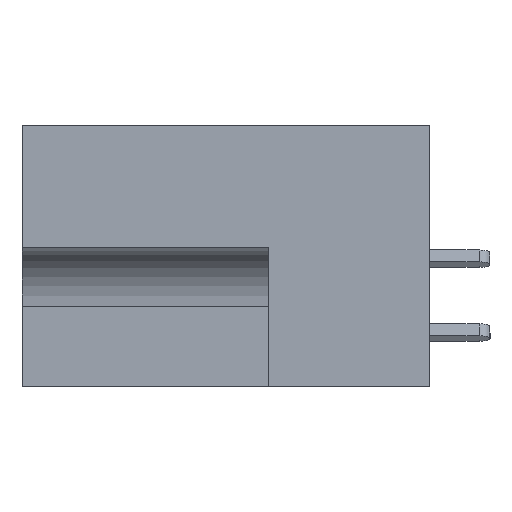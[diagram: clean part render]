
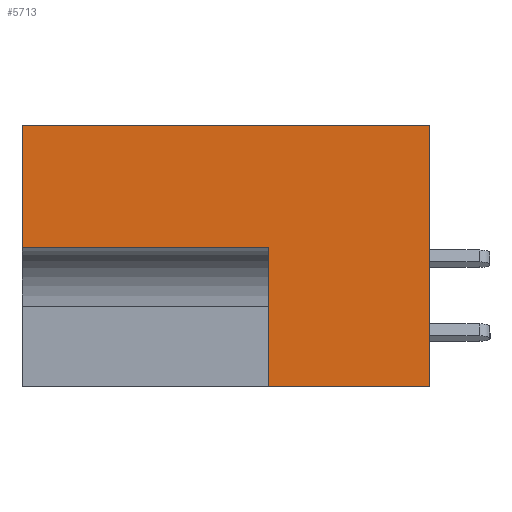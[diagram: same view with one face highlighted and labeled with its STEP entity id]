
A CAD part, left-side view. The second image highlights one B-rep face of the part: STEP entity #5713.
In plain terms, the highlighted planar face has unit normal (-1, 0, 0).
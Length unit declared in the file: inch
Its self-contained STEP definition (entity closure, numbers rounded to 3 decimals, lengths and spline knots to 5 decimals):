
#639 = CARTESIAN_POINT ( 'NONE',  ( 0., 0.453, 0. ) ) ;
#872 = AXIS2_PLACEMENT_3D ( 'NONE', #13198, #6765, #5281 ) ;
#1034 = DIRECTION ( 'NONE',  ( 0., -1., 0. ) ) ;
#1249 = DIRECTION ( 'NONE',  ( 0., 1., 0. ) ) ;
#1355 = ORIENTED_EDGE ( 'NONE', *, *, #11278, .T. ) ;
#2337 = EDGE_CURVE ( 'NONE', #8009, #20477, #3827, .T. ) ;
#2686 = CARTESIAN_POINT ( 'NONE',  ( 0., 0.328, -0.248 ) ) ;
#3179 = VERTEX_POINT ( 'NONE', #6458 ) ;
#3827 = LINE ( 'NONE', #639, #5066 ) ;
#4107 = EDGE_CURVE ( 'NONE', #3179, #8009, #11041, .T. ) ;
#4432 = ORIENTED_EDGE ( 'NONE', *, *, #12451, .F. ) ;
#4786 = EDGE_CURVE ( 'NONE', #13061, #18036, #16835, .T. ) ;
#5066 = VECTOR ( 'NONE', #8846, 39.37008 ) ;
#5281 = DIRECTION ( 'NONE',  ( 0., 0., -1. ) ) ;
#5713 = ADVANCED_FACE ( 'NONE', ( #11478 ), #16769, .F. ) ;
#5969 = VECTOR ( 'NONE', #18970, 39.37008 ) ;
#6180 = CARTESIAN_POINT ( 'NONE',  ( 0., 0.828, 0. ) ) ;
#6458 = CARTESIAN_POINT ( 'NONE',  ( 0., 0.828, -0.248 ) ) ;
#6765 = DIRECTION ( 'NONE',  ( 1., 0., 0. ) ) ;
#6984 = DIRECTION ( 'NONE',  ( 0., 0., 1. ) ) ;
#7018 = CARTESIAN_POINT ( 'NONE',  ( 0., 0., 0. ) ) ;
#7484 = CARTESIAN_POINT ( 'NONE',  ( 0., 0.453, -0.531 ) ) ;
#7502 = LINE ( 'NONE', #19053, #10277 ) ;
#7766 = CARTESIAN_POINT ( 'NONE',  ( 0., 0.328, -0.531 ) ) ;
#8009 = VERTEX_POINT ( 'NONE', #20684 ) ;
#8181 = ORIENTED_EDGE ( 'NONE', *, *, #4786, .F. ) ;
#8846 = DIRECTION ( 'NONE',  ( 0., -1., 0. ) ) ;
#9139 = EDGE_CURVE ( 'NONE', #14839, #20477, #16411, .T. ) ;
#10277 = VECTOR ( 'NONE', #1249, 39.37008 ) ;
#10609 = ORIENTED_EDGE ( 'NONE', *, *, #9139, .T. ) ;
#11041 = LINE ( 'NONE', #6180, #5969 ) ;
#11278 = EDGE_CURVE ( 'NONE', #13061, #14839, #12131, .T. ) ;
#11478 = FACE_OUTER_BOUND ( 'NONE', #19828, .T. ) ;
#12131 = LINE ( 'NONE', #7484, #13376 ) ;
#12451 = EDGE_CURVE ( 'NONE', #18036, #3179, #7502, .T. ) ;
#13061 = VERTEX_POINT ( 'NONE', #7766 ) ;
#13198 = CARTESIAN_POINT ( 'NONE',  ( 0., 0.453, 0. ) ) ;
#13294 = ORIENTED_EDGE ( 'NONE', *, *, #2337, .F. ) ;
#13298 = ORIENTED_EDGE ( 'NONE', *, *, #4107, .F. ) ;
#13376 = VECTOR ( 'NONE', #1034, 39.37008 ) ;
#14839 = VERTEX_POINT ( 'NONE', #19269 ) ;
#15191 = DIRECTION ( 'NONE',  ( 0., 0., 1. ) ) ;
#15830 = VECTOR ( 'NONE', #6984, 39.37008 ) ;
#16411 = LINE ( 'NONE', #18373, #17946 ) ;
#16769 = PLANE ( 'NONE',  #872 ) ;
#16835 = LINE ( 'NONE', #19639, #15830 ) ;
#17946 = VECTOR ( 'NONE', #15191, 39.37008 ) ;
#18036 = VERTEX_POINT ( 'NONE', #2686 ) ;
#18373 = CARTESIAN_POINT ( 'NONE',  ( 0., 0., 0. ) ) ;
#18970 = DIRECTION ( 'NONE',  ( 0., 0., 1. ) ) ;
#19053 = CARTESIAN_POINT ( 'NONE',  ( 0., 0.328, -0.248 ) ) ;
#19269 = CARTESIAN_POINT ( 'NONE',  ( 0., 0., -0.531 ) ) ;
#19639 = CARTESIAN_POINT ( 'NONE',  ( 0., 0.328, -0.531 ) ) ;
#19828 = EDGE_LOOP ( 'NONE', ( #13298, #4432, #8181, #1355, #10609, #13294 ) ) ;
#20477 = VERTEX_POINT ( 'NONE', #7018 ) ;
#20684 = CARTESIAN_POINT ( 'NONE',  ( 0., 0.828, 0. ) ) ;
